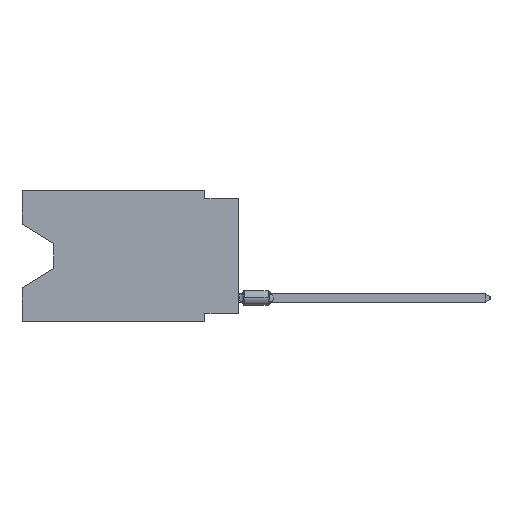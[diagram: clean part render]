
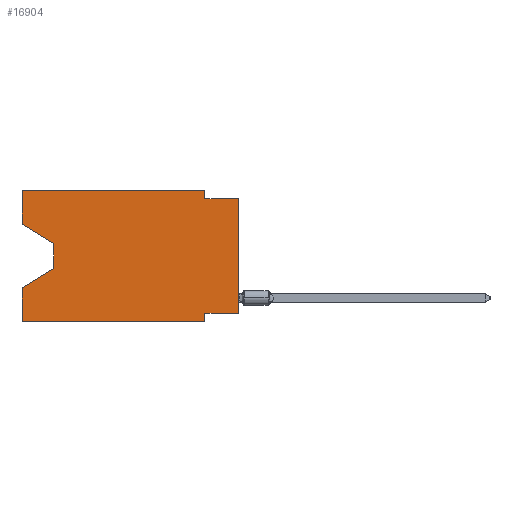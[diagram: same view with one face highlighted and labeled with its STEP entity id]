
A CAD part, left-side view. The second image highlights one B-rep face of the part: STEP entity #16904.
In plain terms, the highlighted planar face has unit normal (-1, 0, 0).
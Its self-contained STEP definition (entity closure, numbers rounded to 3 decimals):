
#46 = DIRECTION ( 'NONE',  ( 0., 0., 1. ) ) ;
#293 = VECTOR ( 'NONE', #27868, 1000. ) ;
#322 = CARTESIAN_POINT ( 'NONE',  ( 0., 0., -0.635 ) ) ;
#850 = DIRECTION ( 'NONE',  ( 0., 0., 1. ) ) ;
#1047 = EDGE_CURVE ( 'NONE', #13755, #4933, #32630, .T. ) ;
#2418 = VECTOR ( 'NONE', #27112, 1000. ) ;
#3252 = LINE ( 'NONE', #6243, #15607 ) ;
#3295 = CARTESIAN_POINT ( 'NONE',  ( 0., 2.54, -9.906 ) ) ;
#3759 = DIRECTION ( 'NONE',  ( 1., 0., 0. ) ) ;
#3994 = ORIENTED_EDGE ( 'NONE', *, *, #17886, .F. ) ;
#4080 = DIRECTION ( 'NONE',  ( 0., -1., 0. ) ) ;
#4098 = VECTOR ( 'NONE', #850, 1000. ) ;
#4533 = DIRECTION ( 'NONE',  ( 0., -1., 0. ) ) ;
#4750 = EDGE_CURVE ( 'NONE', #10012, #21875, #14904, .T. ) ;
#4803 = EDGE_LOOP ( 'NONE', ( #14869, #5494, #12156, #5038, #18532, #3994, #18381, #25605, #20878, #17079, #8880, #18305 ) ) ;
#4933 = VERTEX_POINT ( 'NONE', #21730 ) ;
#5038 = ORIENTED_EDGE ( 'NONE', *, *, #33043, .F. ) ;
#5475 = VECTOR ( 'NONE', #7693, 1000. ) ;
#5494 = ORIENTED_EDGE ( 'NONE', *, *, #29558, .T. ) ;
#6052 = LINE ( 'NONE', #27644, #7385 ) ;
#6124 = CARTESIAN_POINT ( 'NONE',  ( 0., 0., 0. ) ) ;
#6243 = CARTESIAN_POINT ( 'NONE',  ( 0., 2.54, -9.906 ) ) ;
#6424 = DIRECTION ( 'NONE',  ( 0., 0., -1. ) ) ;
#6569 = CARTESIAN_POINT ( 'NONE',  ( 0., 0., -9.271 ) ) ;
#6572 = DIRECTION ( 'NONE',  ( 0., 0., -1. ) ) ;
#6634 = CARTESIAN_POINT ( 'NONE',  ( 0., 13.97, -5.893 ) ) ;
#6749 = CARTESIAN_POINT ( 'NONE',  ( 0., 16.383, 0. ) ) ;
#7075 = LINE ( 'NONE', #20405, #29098 ) ;
#7377 = CARTESIAN_POINT ( 'NONE',  ( 0., 16.383, -9.906 ) ) ;
#7385 = VECTOR ( 'NONE', #6572, 1000. ) ;
#7693 = DIRECTION ( 'NONE',  ( 0., -0.855, -0.519 ) ) ;
#7986 = VERTEX_POINT ( 'NONE', #19980 ) ;
#8880 = ORIENTED_EDGE ( 'NONE', *, *, #4750, .F. ) ;
#9052 = FACE_OUTER_BOUND ( 'NONE', #4803, .T. ) ;
#9987 = CARTESIAN_POINT ( 'NONE',  ( 0., 16.383, 0. ) ) ;
#10012 = VERTEX_POINT ( 'NONE', #34119 ) ;
#10484 = CARTESIAN_POINT ( 'NONE',  ( 0., 13.97, -4.013 ) ) ;
#12156 = ORIENTED_EDGE ( 'NONE', *, *, #29451, .T. ) ;
#12196 = VERTEX_POINT ( 'NONE', #3295 ) ;
#13539 = VECTOR ( 'NONE', #28042, 1000. ) ;
#13755 = VERTEX_POINT ( 'NONE', #21127 ) ;
#13862 = EDGE_CURVE ( 'NONE', #33927, #4933, #21931, .T. ) ;
#14247 = CARTESIAN_POINT ( 'NONE',  ( 0., 2.54, -9.271 ) ) ;
#14869 = ORIENTED_EDGE ( 'NONE', *, *, #32076, .T. ) ;
#14904 = LINE ( 'NONE', #9987, #24184 ) ;
#15085 = VECTOR ( 'NONE', #46, 1000. ) ;
#15261 = CARTESIAN_POINT ( 'NONE',  ( 0., 16.383, -2.546 ) ) ;
#15294 = CARTESIAN_POINT ( 'NONE',  ( 0., 13.97, -5.893 ) ) ;
#15551 = AXIS2_PLACEMENT_3D ( 'NONE', #6749, #3759, #33624 ) ;
#15607 = VECTOR ( 'NONE', #6424, 1000. ) ;
#16286 = LINE ( 'NONE', #26996, #5475 ) ;
#16904 = ADVANCED_FACE ( 'NONE', ( #9052 ), #27830, .F. ) ;
#17079 = ORIENTED_EDGE ( 'NONE', *, *, #22895, .F. ) ;
#17151 = CARTESIAN_POINT ( 'NONE',  ( 0., 13.97, -4.013 ) ) ;
#17269 = CARTESIAN_POINT ( 'NONE',  ( 0., 2.54, 0. ) ) ;
#17886 = EDGE_CURVE ( 'NONE', #23175, #12196, #3252, .T. ) ;
#18305 = ORIENTED_EDGE ( 'NONE', *, *, #24819, .F. ) ;
#18381 = ORIENTED_EDGE ( 'NONE', *, *, #24307, .F. ) ;
#18532 = ORIENTED_EDGE ( 'NONE', *, *, #32758, .T. ) ;
#18998 = LINE ( 'NONE', #24626, #15085 ) ;
#19980 = CARTESIAN_POINT ( 'NONE',  ( 0., 16.383, -7.36 ) ) ;
#20405 = CARTESIAN_POINT ( 'NONE',  ( 0., 16.383, -9.906 ) ) ;
#20848 = CARTESIAN_POINT ( 'NONE',  ( 0., 0., -9.271 ) ) ;
#20878 = ORIENTED_EDGE ( 'NONE', *, *, #1047, .F. ) ;
#21127 = CARTESIAN_POINT ( 'NONE',  ( 0., 2.54, -0.635 ) ) ;
#21401 = VERTEX_POINT ( 'NONE', #17151 ) ;
#21730 = CARTESIAN_POINT ( 'NONE',  ( 0., 0., -0.635 ) ) ;
#21875 = VERTEX_POINT ( 'NONE', #17269 ) ;
#21931 = LINE ( 'NONE', #6124, #4098 ) ;
#22895 = EDGE_CURVE ( 'NONE', #21875, #13755, #6052, .T. ) ;
#23175 = VERTEX_POINT ( 'NONE', #14247 ) ;
#23704 = VECTOR ( 'NONE', #31577, 1000. ) ;
#24143 = LINE ( 'NONE', #29747, #2418 ) ;
#24184 = VECTOR ( 'NONE', #4533, 1000. ) ;
#24307 = EDGE_CURVE ( 'NONE', #33927, #23175, #34207, .T. ) ;
#24626 = CARTESIAN_POINT ( 'NONE',  ( 0., 16.383, 0. ) ) ;
#24819 = EDGE_CURVE ( 'NONE', #30708, #10012, #24143, .T. ) ;
#25605 = ORIENTED_EDGE ( 'NONE', *, *, #13862, .T. ) ;
#26537 = VERTEX_POINT ( 'NONE', #15294 ) ;
#26996 = CARTESIAN_POINT ( 'NONE',  ( 0., 16.383, -2.546 ) ) ;
#27112 = DIRECTION ( 'NONE',  ( 0., 0., 1. ) ) ;
#27339 = VECTOR ( 'NONE', #34022, 1000. ) ;
#27644 = CARTESIAN_POINT ( 'NONE',  ( 0., 2.54, 0. ) ) ;
#27830 = PLANE ( 'NONE',  #15551 ) ;
#27868 = DIRECTION ( 'NONE',  ( 0., -1., 0. ) ) ;
#28042 = DIRECTION ( 'NONE',  ( 0., 0.855, -0.519 ) ) ;
#29098 = VECTOR ( 'NONE', #4080, 1000. ) ;
#29451 = EDGE_CURVE ( 'NONE', #26537, #7986, #33496, .T. ) ;
#29558 = EDGE_CURVE ( 'NONE', #21401, #26537, #34366, .T. ) ;
#29747 = CARTESIAN_POINT ( 'NONE',  ( 0., 16.383, 0. ) ) ;
#30708 = VERTEX_POINT ( 'NONE', #15261 ) ;
#31509 = VERTEX_POINT ( 'NONE', #7377 ) ;
#31577 = DIRECTION ( 'NONE',  ( 0., 1., 0. ) ) ;
#32076 = EDGE_CURVE ( 'NONE', #30708, #21401, #16286, .T. ) ;
#32630 = LINE ( 'NONE', #322, #293 ) ;
#32758 = EDGE_CURVE ( 'NONE', #31509, #12196, #7075, .T. ) ;
#33043 = EDGE_CURVE ( 'NONE', #31509, #7986, #18998, .T. ) ;
#33496 = LINE ( 'NONE', #6634, #13539 ) ;
#33624 = DIRECTION ( 'NONE',  ( 0., 0., -1. ) ) ;
#33927 = VERTEX_POINT ( 'NONE', #6569 ) ;
#34022 = DIRECTION ( 'NONE',  ( 0., 0., -1. ) ) ;
#34119 = CARTESIAN_POINT ( 'NONE',  ( 0., 16.383, 0. ) ) ;
#34207 = LINE ( 'NONE', #20848, #23704 ) ;
#34366 = LINE ( 'NONE', #10484, #27339 ) ;
